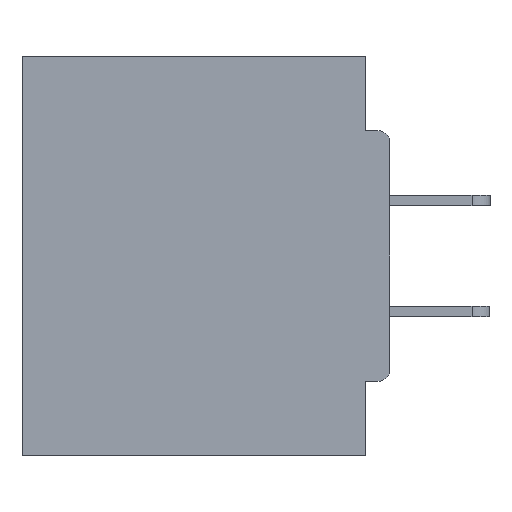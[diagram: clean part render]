
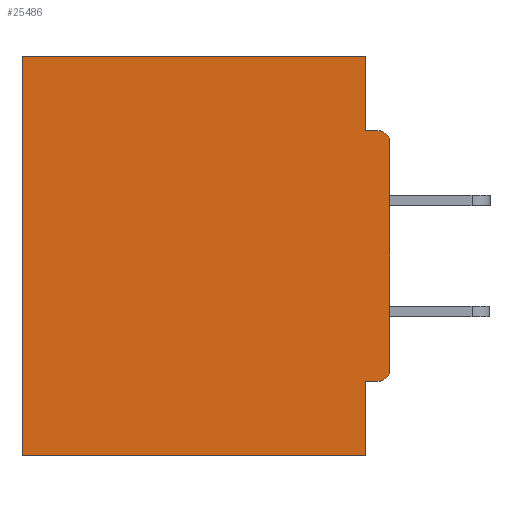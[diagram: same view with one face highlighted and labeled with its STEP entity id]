
A CAD part, left-side view. The second image highlights one B-rep face of the part: STEP entity #25486.
In plain terms, the highlighted planar face has unit normal (-1, 0, 0).
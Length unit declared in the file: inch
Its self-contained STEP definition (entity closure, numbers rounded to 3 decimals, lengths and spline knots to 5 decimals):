
#215 = AXIS2_PLACEMENT_3D ( 'NONE', #1505, #9032, #1400 ) ;
#557 = DIRECTION ( 'NONE',  ( 0., 1., 0. ) ) ;
#1021 = EDGE_CURVE ( 'NONE', #4944, #16104, #12554, .T. ) ;
#1126 = ORIENTED_EDGE ( 'NONE', *, *, #23445, .T. ) ;
#1171 = AXIS2_PLACEMENT_3D ( 'NONE', #7024, #22381, #14673 ) ;
#1400 = DIRECTION ( 'NONE',  ( 0., 0., -1. ) ) ;
#1505 = CARTESIAN_POINT ( 'NONE',  ( 0.298, 0.015, -0.1085 ) ) ;
#1761 = CIRCLE ( 'NONE', #1171, 0.015 ) ;
#2211 = CARTESIAN_POINT ( 'NONE',  ( 0.298, 0., 0. ) ) ;
#2308 = VECTOR ( 'NONE', #5080, 39.37008 ) ;
#3346 = VECTOR ( 'NONE', #557, 39.37008 ) ;
#3562 = VECTOR ( 'NONE', #20756, 39.37008 ) ;
#3779 = EDGE_CURVE ( 'NONE', #30410, #3835, #15609, .T. ) ;
#3835 = VERTEX_POINT ( 'NONE', #12182 ) ;
#3952 = EDGE_CURVE ( 'NONE', #11585, #3835, #10066, .T. ) ;
#4393 = ORIENTED_EDGE ( 'NONE', *, *, #29583, .F. ) ;
#4632 = DIRECTION ( 'NONE',  ( 0., 0., -1. ) ) ;
#4944 = VERTEX_POINT ( 'NONE', #18488 ) ;
#4953 = DIRECTION ( 'NONE',  ( 0., 1., 0. ) ) ;
#5080 = DIRECTION ( 'NONE',  ( 0., 0., -1. ) ) ;
#5811 = CARTESIAN_POINT ( 'NONE',  ( 0.298, 0., -0.0935 ) ) ;
#6407 = LINE ( 'NONE', #10397, #3346 ) ;
#7024 = CARTESIAN_POINT ( 'NONE',  ( 0.298, 0.015, -0.3915 ) ) ;
#8085 = VECTOR ( 'NONE', #10053, 39.37008 ) ;
#8447 = VECTOR ( 'NONE', #17998, 39.37008 ) ;
#9032 = DIRECTION ( 'NONE',  ( -1., 0., 0. ) ) ;
#10053 = DIRECTION ( 'NONE',  ( 0., -1., 0. ) ) ;
#10066 = CIRCLE ( 'NONE', #215, 0.015 ) ;
#10397 = CARTESIAN_POINT ( 'NONE',  ( 0.298, 0., -0.5 ) ) ;
#11537 = CARTESIAN_POINT ( 'NONE',  ( 0.298, 0.031, -0.4065 ) ) ;
#11585 = VERTEX_POINT ( 'NONE', #30486 ) ;
#11917 = DIRECTION ( 'NONE',  ( 0., 0., -1. ) ) ;
#12143 = ORIENTED_EDGE ( 'NONE', *, *, #19383, .F. ) ;
#12182 = CARTESIAN_POINT ( 'NONE',  ( 0.298, 0.015, -0.0935 ) ) ;
#12554 = LINE ( 'NONE', #17455, #29923 ) ;
#13477 = CARTESIAN_POINT ( 'NONE',  ( 0.298, 0.46, 0. ) ) ;
#13687 = EDGE_CURVE ( 'NONE', #26536, #30410, #14915, .T. ) ;
#14022 = FACE_OUTER_BOUND ( 'NONE', #17508, .T. ) ;
#14084 = LINE ( 'NONE', #17999, #2308 ) ;
#14256 = CARTESIAN_POINT ( 'NONE',  ( 0.298, 0.031, -0.0935 ) ) ;
#14673 = DIRECTION ( 'NONE',  ( 0., 0., -1. ) ) ;
#14718 = EDGE_CURVE ( 'NONE', #29350, #20937, #28584, .T. ) ;
#14915 = LINE ( 'NONE', #24357, #19234 ) ;
#15496 = VERTEX_POINT ( 'NONE', #25390 ) ;
#15609 = LINE ( 'NONE', #5811, #8085 ) ;
#15736 = EDGE_CURVE ( 'NONE', #4944, #16720, #1761, .T. ) ;
#16104 = VERTEX_POINT ( 'NONE', #11537 ) ;
#16720 = VERTEX_POINT ( 'NONE', #30952 ) ;
#16727 = CARTESIAN_POINT ( 'NONE',  ( 0.298, 0.46, 0. ) ) ;
#17455 = CARTESIAN_POINT ( 'NONE',  ( 0.298, 0., -0.4065 ) ) ;
#17508 = EDGE_LOOP ( 'NONE', ( #30826, #21377, #25536, #1126, #30531, #4393, #22062, #31640, #32095, #12143 ) ) ;
#17998 = DIRECTION ( 'NONE',  ( 0., 0., -1. ) ) ;
#17999 = CARTESIAN_POINT ( 'NONE',  ( 0.298, 0.031, -0.5 ) ) ;
#18488 = CARTESIAN_POINT ( 'NONE',  ( 0.298, 0.015, -0.4065 ) ) ;
#19234 = VECTOR ( 'NONE', #11917, 39.37008 ) ;
#19383 = EDGE_CURVE ( 'NONE', #11585, #16720, #24361, .T. ) ;
#19775 = EDGE_CURVE ( 'NONE', #16104, #15496, #14084, .T. ) ;
#19782 = DIRECTION ( 'NONE',  ( 1., 0., 0. ) ) ;
#20458 = LINE ( 'NONE', #28049, #3562 ) ;
#20756 = DIRECTION ( 'NONE',  ( 0., 1., 0. ) ) ;
#20937 = VERTEX_POINT ( 'NONE', #29122 ) ;
#21374 = CARTESIAN_POINT ( 'NONE',  ( 0.298, 0.031, 0. ) ) ;
#21377 = ORIENTED_EDGE ( 'NONE', *, *, #3779, .F. ) ;
#22062 = ORIENTED_EDGE ( 'NONE', *, *, #19775, .F. ) ;
#22381 = DIRECTION ( 'NONE',  ( -1., 0., 0. ) ) ;
#23445 = EDGE_CURVE ( 'NONE', #26536, #29350, #20458, .T. ) ;
#24357 = CARTESIAN_POINT ( 'NONE',  ( 0.298, 0.031, -0.5 ) ) ;
#24361 = LINE ( 'NONE', #25251, #29902 ) ;
#25251 = CARTESIAN_POINT ( 'NONE',  ( 0.298, 0., 0. ) ) ;
#25390 = CARTESIAN_POINT ( 'NONE',  ( 0.298, 0.031, -0.5 ) ) ;
#25486 = ADVANCED_FACE ( 'NONE', ( #14022 ), #30035, .F. ) ;
#25536 = ORIENTED_EDGE ( 'NONE', *, *, #13687, .F. ) ;
#26055 = AXIS2_PLACEMENT_3D ( 'NONE', #2211, #19782, #32540 ) ;
#26536 = VERTEX_POINT ( 'NONE', #21374 ) ;
#28049 = CARTESIAN_POINT ( 'NONE',  ( 0.298, 0., 0. ) ) ;
#28584 = LINE ( 'NONE', #13477, #8447 ) ;
#29122 = CARTESIAN_POINT ( 'NONE',  ( 0.298, 0.46, -0.5 ) ) ;
#29350 = VERTEX_POINT ( 'NONE', #16727 ) ;
#29583 = EDGE_CURVE ( 'NONE', #15496, #20937, #6407, .T. ) ;
#29902 = VECTOR ( 'NONE', #4632, 39.37008 ) ;
#29923 = VECTOR ( 'NONE', #4953, 39.37008 ) ;
#30035 = PLANE ( 'NONE',  #26055 ) ;
#30410 = VERTEX_POINT ( 'NONE', #14256 ) ;
#30486 = CARTESIAN_POINT ( 'NONE',  ( 0.298, 0., -0.1085 ) ) ;
#30531 = ORIENTED_EDGE ( 'NONE', *, *, #14718, .T. ) ;
#30826 = ORIENTED_EDGE ( 'NONE', *, *, #3952, .T. ) ;
#30952 = CARTESIAN_POINT ( 'NONE',  ( 0.298, 0., -0.3915 ) ) ;
#31640 = ORIENTED_EDGE ( 'NONE', *, *, #1021, .F. ) ;
#32095 = ORIENTED_EDGE ( 'NONE', *, *, #15736, .T. ) ;
#32540 = DIRECTION ( 'NONE',  ( 0., 0., -1. ) ) ;
